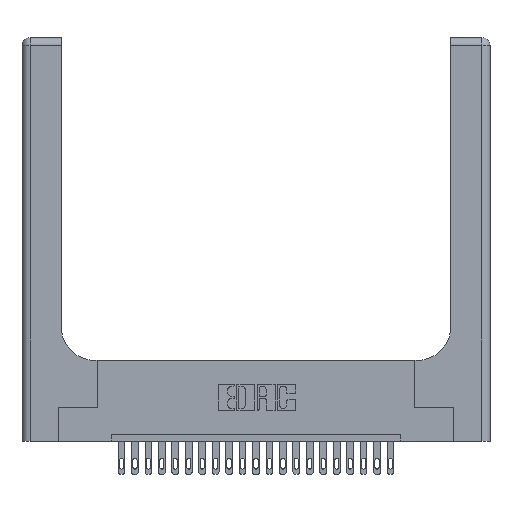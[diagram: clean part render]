
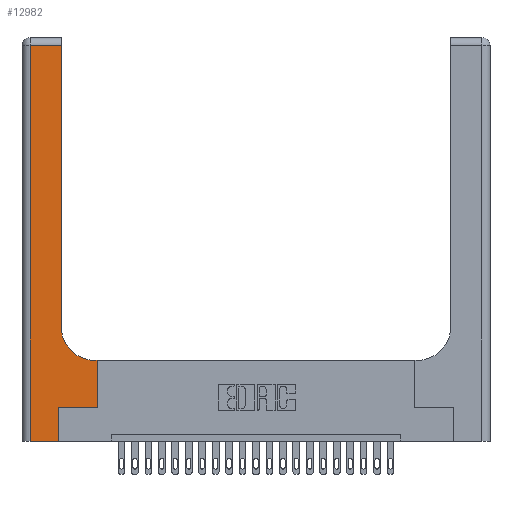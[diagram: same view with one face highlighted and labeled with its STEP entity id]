
A CAD part, top view. The second image highlights one B-rep face of the part: STEP entity #12982.
In plain terms, the highlighted planar face has unit normal (0, 0, 1).
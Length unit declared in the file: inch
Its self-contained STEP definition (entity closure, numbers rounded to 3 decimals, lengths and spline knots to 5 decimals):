
#138 = VERTEX_POINT ( 'NONE', #11143 ) ;
#205 = DIRECTION ( 'NONE',  ( 0., -1., 0. ) ) ;
#309 = EDGE_CURVE ( 'NONE', #19041, #138, #22383, .T. ) ;
#1118 = VECTOR ( 'NONE', #2649, 39.37008 ) ;
#1493 = VERTEX_POINT ( 'NONE', #9979 ) ;
#1528 = DIRECTION ( 'NONE',  ( 1., 0., 0. ) ) ;
#1742 = EDGE_CURVE ( 'NONE', #1493, #19650, #12640, .T. ) ;
#2493 = CARTESIAN_POINT ( 'NONE',  ( 0.06, 0., 0.37 ) ) ;
#2576 = EDGE_CURVE ( 'NONE', #138, #17159, #23597, .T. ) ;
#2649 = DIRECTION ( 'NONE',  ( 0., 1., 0. ) ) ;
#2976 = DIRECTION ( 'NONE',  ( 1., 0., 0. ) ) ;
#3069 = DIRECTION ( 'NONE',  ( -1., 0., 0. ) ) ;
#3345 = VERTEX_POINT ( 'NONE', #6780 ) ;
#3758 = EDGE_CURVE ( 'NONE', #6137, #3345, #18633, .T. ) ;
#4040 = LINE ( 'NONE', #10756, #8065 ) ;
#4961 = AXIS2_PLACEMENT_3D ( 'NONE', #8712, #12315, #12402 ) ;
#5043 = CARTESIAN_POINT ( 'NONE',  ( 0.06, 2.94, 0.37 ) ) ;
#5236 = VECTOR ( 'NONE', #17248, 39.37008 ) ;
#5254 = CARTESIAN_POINT ( 'NONE',  ( 0.5585, 0.25, 0.37 ) ) ;
#5271 = ORIENTED_EDGE ( 'NONE', *, *, #3758, .T. ) ;
#5711 = CARTESIAN_POINT ( 'NONE',  ( 0., 3., 0.37 ) ) ;
#6137 = VERTEX_POINT ( 'NONE', #2493 ) ;
#6215 = CARTESIAN_POINT ( 'NONE',  ( 0.2915, 0.6, 0.37 ) ) ;
#6780 = CARTESIAN_POINT ( 'NONE',  ( 0.269, 0., 0.37 ) ) ;
#6833 = CARTESIAN_POINT ( 'NONE',  ( 0., 0., 0.37 ) ) ;
#7559 = EDGE_CURVE ( 'NONE', #11145, #19041, #16786, .T. ) ;
#7728 = VECTOR ( 'NONE', #1528, 39.37008 ) ;
#8065 = VECTOR ( 'NONE', #10590, 39.37008 ) ;
#8712 = CARTESIAN_POINT ( 'NONE',  ( 0.5415, 0.85, 0.37 ) ) ;
#8782 = ORIENTED_EDGE ( 'NONE', *, *, #11337, .T. ) ;
#8786 = CARTESIAN_POINT ( 'NONE',  ( 0., 2.94, 0.37 ) ) ;
#9785 = CARTESIAN_POINT ( 'NONE',  ( 0.5585, 0.6, 0.37 ) ) ;
#9970 = LINE ( 'NONE', #11380, #17100 ) ;
#9979 = CARTESIAN_POINT ( 'NONE',  ( 0.269, 0.25, 0.37 ) ) ;
#10590 = DIRECTION ( 'NONE',  ( 0., 1., 0. ) ) ;
#10756 = CARTESIAN_POINT ( 'NONE',  ( 0.5585, 0.25, 0.37 ) ) ;
#10980 = LINE ( 'NONE', #6215, #20621 ) ;
#11143 = CARTESIAN_POINT ( 'NONE',  ( 0.2915, 2.94, 0.37 ) ) ;
#11145 = VERTEX_POINT ( 'NONE', #17255 ) ;
#11337 = EDGE_CURVE ( 'NONE', #17159, #6137, #9970, .T. ) ;
#11360 = AXIS2_PLACEMENT_3D ( 'NONE', #5711, #18503, #17703 ) ;
#11380 = CARTESIAN_POINT ( 'NONE',  ( 0.06, 3., 0.37 ) ) ;
#11406 = ORIENTED_EDGE ( 'NONE', *, *, #309, .T. ) ;
#12162 = CARTESIAN_POINT ( 'NONE',  ( 0.2915, 0.85, 0.37 ) ) ;
#12315 = DIRECTION ( 'NONE',  ( 0., 0., -1. ) ) ;
#12402 = DIRECTION ( 'NONE',  ( 1., 0., 0. ) ) ;
#12640 = LINE ( 'NONE', #14042, #7728 ) ;
#12982 = ADVANCED_FACE ( 'NONE', ( #22159 ), #18803, .F. ) ;
#13158 = ORIENTED_EDGE ( 'NONE', *, *, #22775, .T. ) ;
#13416 = ORIENTED_EDGE ( 'NONE', *, *, #1742, .T. ) ;
#13489 = CARTESIAN_POINT ( 'NONE',  ( 0.269, 0., 0.37 ) ) ;
#13753 = ORIENTED_EDGE ( 'NONE', *, *, #7559, .T. ) ;
#14042 = CARTESIAN_POINT ( 'NONE',  ( 0.269, 0.25, 0.37 ) ) ;
#16039 = LINE ( 'NONE', #13489, #1118 ) ;
#16258 = ORIENTED_EDGE ( 'NONE', *, *, #22203, .T. ) ;
#16786 = CIRCLE ( 'NONE', #4961, 0.25 ) ;
#17100 = VECTOR ( 'NONE', #205, 39.37008 ) ;
#17159 = VERTEX_POINT ( 'NONE', #5043 ) ;
#17248 = DIRECTION ( 'NONE',  ( 0., 1., 0. ) ) ;
#17255 = CARTESIAN_POINT ( 'NONE',  ( 0.5415, 0.6, 0.37 ) ) ;
#17703 = DIRECTION ( 'NONE',  ( -1., 0., 0. ) ) ;
#17975 = EDGE_LOOP ( 'NONE', ( #11406, #21225, #8782, #5271, #23673, #13416, #13158, #16258, #13753 ) ) ;
#18503 = DIRECTION ( 'NONE',  ( 0., 0., -1. ) ) ;
#18633 = LINE ( 'NONE', #6833, #21776 ) ;
#18803 = PLANE ( 'NONE',  #11360 ) ;
#18976 = VECTOR ( 'NONE', #3069, 39.37008 ) ;
#19041 = VERTEX_POINT ( 'NONE', #12162 ) ;
#19393 = DIRECTION ( 'NONE',  ( -1., 0., 0. ) ) ;
#19650 = VERTEX_POINT ( 'NONE', #5254 ) ;
#20390 = VERTEX_POINT ( 'NONE', #9785 ) ;
#20621 = VECTOR ( 'NONE', #19393, 39.37008 ) ;
#21066 = EDGE_CURVE ( 'NONE', #3345, #1493, #16039, .T. ) ;
#21225 = ORIENTED_EDGE ( 'NONE', *, *, #2576, .T. ) ;
#21776 = VECTOR ( 'NONE', #2976, 39.37008 ) ;
#22159 = FACE_OUTER_BOUND ( 'NONE', #17975, .T. ) ;
#22203 = EDGE_CURVE ( 'NONE', #20390, #11145, #10980, .T. ) ;
#22383 = LINE ( 'NONE', #22675, #5236 ) ;
#22675 = CARTESIAN_POINT ( 'NONE',  ( 0.2915, 3., 0.37 ) ) ;
#22775 = EDGE_CURVE ( 'NONE', #19650, #20390, #4040, .T. ) ;
#23597 = LINE ( 'NONE', #8786, #18976 ) ;
#23673 = ORIENTED_EDGE ( 'NONE', *, *, #21066, .T. ) ;
